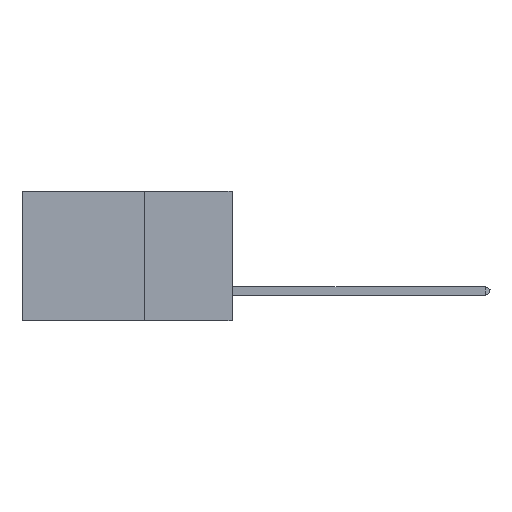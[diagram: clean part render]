
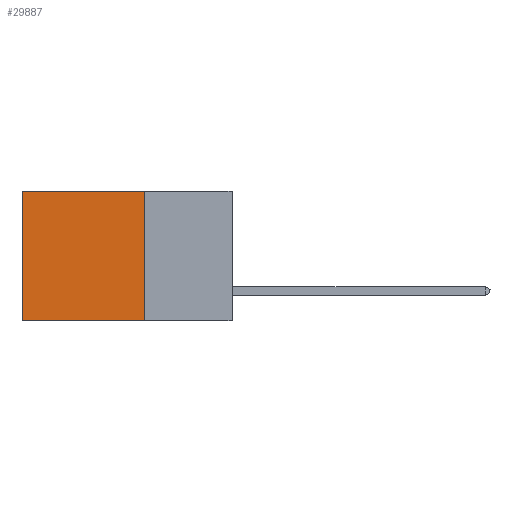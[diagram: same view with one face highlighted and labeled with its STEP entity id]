
A CAD part, left-side view. The second image highlights one B-rep face of the part: STEP entity #29887.
In plain terms, the highlighted planar face has unit normal (-1, 0, 0).
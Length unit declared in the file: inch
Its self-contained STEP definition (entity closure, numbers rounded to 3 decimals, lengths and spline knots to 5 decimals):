
#2064 = CARTESIAN_POINT ( 'NONE',  ( 0.2875, 0.25, 0. ) ) ;
#3044 = CARTESIAN_POINT ( 'NONE',  ( 0.2875, 0.25, -0.37 ) ) ;
#4247 = ORIENTED_EDGE ( 'NONE', *, *, #15548, .F. ) ;
#4780 = CARTESIAN_POINT ( 'NONE',  ( 0.2875, 0.6, 0. ) ) ;
#5530 = CARTESIAN_POINT ( 'NONE',  ( 0.2875, 0.6, -0.37 ) ) ;
#5860 = ORIENTED_EDGE ( 'NONE', *, *, #15326, .T. ) ;
#7014 = ORIENTED_EDGE ( 'NONE', *, *, #19245, .T. ) ;
#9055 = VECTOR ( 'NONE', #20923, 39.37008 ) ;
#9198 = CARTESIAN_POINT ( 'NONE',  ( 0.2875, 0.25, 0. ) ) ;
#10690 = CARTESIAN_POINT ( 'NONE',  ( 0.2875, 0.25, 0. ) ) ;
#11524 = AXIS2_PLACEMENT_3D ( 'NONE', #2064, #30227, #23071 ) ;
#11922 = CARTESIAN_POINT ( 'NONE',  ( 0.2875, 0.25, 0. ) ) ;
#13117 = EDGE_CURVE ( 'NONE', #30804, #23891, #21308, .T. ) ;
#15326 = EDGE_CURVE ( 'NONE', #30804, #28081, #22311, .T. ) ;
#15397 = LINE ( 'NONE', #20566, #20231 ) ;
#15548 = EDGE_CURVE ( 'NONE', #23891, #21322, #25984, .T. ) ;
#16200 = DIRECTION ( 'NONE',  ( 0., 0., -1. ) ) ;
#16388 = DIRECTION ( 'NONE',  ( 0., 1., 0. ) ) ;
#17553 = DIRECTION ( 'NONE',  ( 0., 1., 0. ) ) ;
#19245 = EDGE_CURVE ( 'NONE', #28081, #21322, #15397, .T. ) ;
#20192 = EDGE_LOOP ( 'NONE', ( #7014, #4247, #24848, #5860 ) ) ;
#20231 = VECTOR ( 'NONE', #16200, 39.37008 ) ;
#20566 = CARTESIAN_POINT ( 'NONE',  ( 0.2875, 0.6, 0. ) ) ;
#20923 = DIRECTION ( 'NONE',  ( 0., 0., -1. ) ) ;
#21195 = VECTOR ( 'NONE', #16388, 39.37008 ) ;
#21308 = LINE ( 'NONE', #9198, #9055 ) ;
#21322 = VERTEX_POINT ( 'NONE', #5530 ) ;
#22128 = FACE_OUTER_BOUND ( 'NONE', #20192, .T. ) ;
#22311 = LINE ( 'NONE', #10690, #23052 ) ;
#23052 = VECTOR ( 'NONE', #17553, 39.37008 ) ;
#23071 = DIRECTION ( 'NONE',  ( 0., 0., -1. ) ) ;
#23891 = VERTEX_POINT ( 'NONE', #3044 ) ;
#24848 = ORIENTED_EDGE ( 'NONE', *, *, #13117, .F. ) ;
#25984 = LINE ( 'NONE', #28113, #21195 ) ;
#28081 = VERTEX_POINT ( 'NONE', #4780 ) ;
#28113 = CARTESIAN_POINT ( 'NONE',  ( 0.2875, 0.25, -0.37 ) ) ;
#28239 = PLANE ( 'NONE',  #11524 ) ;
#29887 = ADVANCED_FACE ( 'NONE', ( #22128 ), #28239, .F. ) ;
#30227 = DIRECTION ( 'NONE',  ( 1., 0., 0. ) ) ;
#30804 = VERTEX_POINT ( 'NONE', #11922 ) ;
